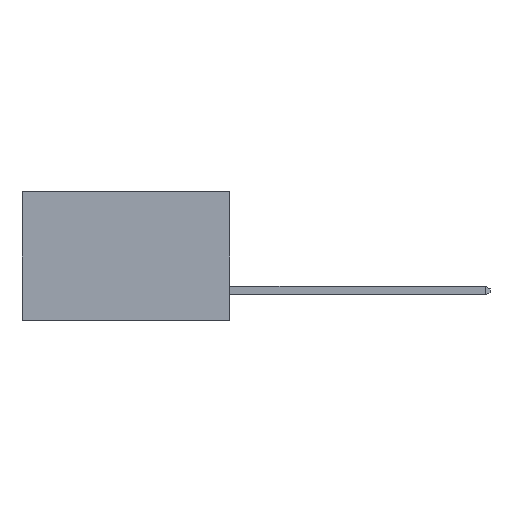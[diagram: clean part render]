
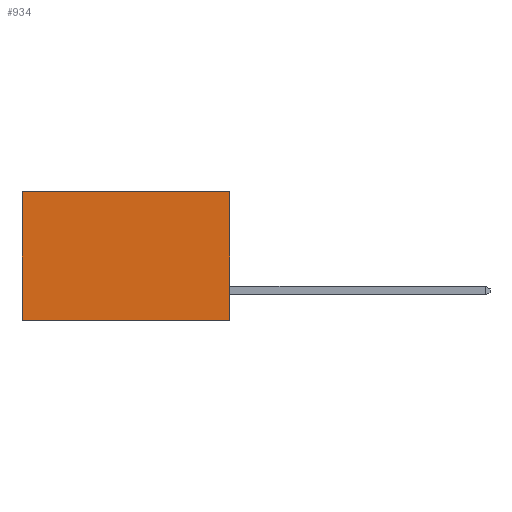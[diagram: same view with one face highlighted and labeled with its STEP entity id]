
A CAD part, left-side view. The second image highlights one B-rep face of the part: STEP entity #934.
In plain terms, the highlighted planar face has unit normal (-1, 0, 0).
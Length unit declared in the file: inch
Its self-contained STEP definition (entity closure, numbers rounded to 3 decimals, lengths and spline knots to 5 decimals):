
#339 = EDGE_LOOP ( 'NONE', ( #4957, #3922, #12264, #594 ) ) ;
#471 = EDGE_CURVE ( 'NONE', #3331, #11758, #4636, .T. ) ;
#594 = ORIENTED_EDGE ( 'NONE', *, *, #5657, .T. ) ;
#916 = PLANE ( 'NONE',  #8290 ) ;
#934 = ADVANCED_FACE ( 'NONE', ( #10081 ), #916, .F. ) ;
#1433 = EDGE_CURVE ( 'NONE', #1886, #10532, #2407, .T. ) ;
#1800 = LINE ( 'NONE', #12691, #11369 ) ;
#1886 = VERTEX_POINT ( 'NONE', #7008 ) ;
#2407 = LINE ( 'NONE', #10139, #11982 ) ;
#2523 = CARTESIAN_POINT ( 'NONE',  ( 0.2615, 0.6, -0.37 ) ) ;
#3031 = DIRECTION ( 'NONE',  ( 0., 0., -1. ) ) ;
#3107 = CARTESIAN_POINT ( 'NONE',  ( 0.2615, 0., 0. ) ) ;
#3331 = VERTEX_POINT ( 'NONE', #10912 ) ;
#3597 = EDGE_CURVE ( 'NONE', #11758, #10532, #1800, .T. ) ;
#3922 = ORIENTED_EDGE ( 'NONE', *, *, #3597, .F. ) ;
#4636 = LINE ( 'NONE', #5022, #6059 ) ;
#4957 = ORIENTED_EDGE ( 'NONE', *, *, #1433, .T. ) ;
#5022 = CARTESIAN_POINT ( 'NONE',  ( 0.2615, 0., -0.37 ) ) ;
#5657 = EDGE_CURVE ( 'NONE', #3331, #1886, #9556, .T. ) ;
#6059 = VECTOR ( 'NONE', #12196, 39.37008 ) ;
#6780 = VECTOR ( 'NONE', #7101, 39.37008 ) ;
#7008 = CARTESIAN_POINT ( 'NONE',  ( 0.2615, 0.6, 0. ) ) ;
#7101 = DIRECTION ( 'NONE',  ( 0., 1., 0. ) ) ;
#8290 = AXIS2_PLACEMENT_3D ( 'NONE', #13183, #12133, #11153 ) ;
#9556 = LINE ( 'NONE', #3107, #6780 ) ;
#10081 = FACE_OUTER_BOUND ( 'NONE', #339, .T. ) ;
#10139 = CARTESIAN_POINT ( 'NONE',  ( 0.2615, 0.6, -0.37 ) ) ;
#10532 = VERTEX_POINT ( 'NONE', #2523 ) ;
#10704 = DIRECTION ( 'NONE',  ( 0., 1., 0. ) ) ;
#10912 = CARTESIAN_POINT ( 'NONE',  ( 0.2615, 0., 0. ) ) ;
#11071 = CARTESIAN_POINT ( 'NONE',  ( 0.2615, 0., -0.37 ) ) ;
#11153 = DIRECTION ( 'NONE',  ( 0., 0., -1. ) ) ;
#11369 = VECTOR ( 'NONE', #10704, 39.37008 ) ;
#11758 = VERTEX_POINT ( 'NONE', #11071 ) ;
#11982 = VECTOR ( 'NONE', #3031, 39.37008 ) ;
#12133 = DIRECTION ( 'NONE',  ( 1., 0., 0. ) ) ;
#12196 = DIRECTION ( 'NONE',  ( 0., 0., -1. ) ) ;
#12264 = ORIENTED_EDGE ( 'NONE', *, *, #471, .F. ) ;
#12691 = CARTESIAN_POINT ( 'NONE',  ( 0.2615, 0., -0.37 ) ) ;
#13183 = CARTESIAN_POINT ( 'NONE',  ( 0.2615, 0., -0.37 ) ) ;
